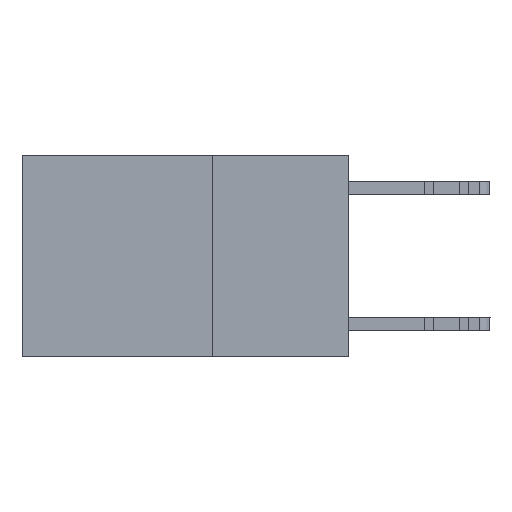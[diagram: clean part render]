
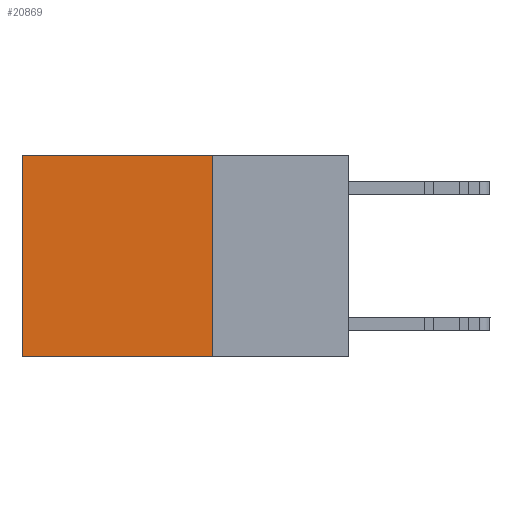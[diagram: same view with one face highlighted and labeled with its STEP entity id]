
A CAD part, left-side view. The second image highlights one B-rep face of the part: STEP entity #20869.
In plain terms, the highlighted planar face has unit normal (-1, 0, 0).
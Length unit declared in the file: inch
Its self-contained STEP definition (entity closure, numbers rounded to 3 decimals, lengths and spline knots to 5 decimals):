
#2307 = DIRECTION ( 'NONE',  ( 0., 0., -1. ) ) ;
#2940 = VECTOR ( 'NONE', #20422, 39.37008 ) ;
#3790 = LINE ( 'NONE', #25389, #2940 ) ;
#4039 = EDGE_CURVE ( 'NONE', #20741, #28897, #4677, .T. ) ;
#4332 = VECTOR ( 'NONE', #23556, 39.37008 ) ;
#4677 = LINE ( 'NONE', #25523, #4332 ) ;
#5005 = CARTESIAN_POINT ( 'NONE',  ( 0.2625, 0.6, -0.37 ) ) ;
#5648 = ORIENTED_EDGE ( 'NONE', *, *, #29035, .T. ) ;
#5797 = EDGE_CURVE ( 'NONE', #12769, #15452, #21283, .T. ) ;
#6502 = CARTESIAN_POINT ( 'NONE',  ( 0.2625, 0.25, 0. ) ) ;
#7311 = DIRECTION ( 'NONE',  ( 0., 0., -1. ) ) ;
#7566 = CARTESIAN_POINT ( 'NONE',  ( 0.2625, 0.25, 0. ) ) ;
#8983 = EDGE_CURVE ( 'NONE', #15452, #28897, #22191, .T. ) ;
#11706 = FACE_OUTER_BOUND ( 'NONE', #30115, .T. ) ;
#12769 = VERTEX_POINT ( 'NONE', #6502 ) ;
#14341 = CARTESIAN_POINT ( 'NONE',  ( 0.2625, 0.6, 0. ) ) ;
#14862 = DIRECTION ( 'NONE',  ( 0., 1., 0. ) ) ;
#14876 = PLANE ( 'NONE',  #24921 ) ;
#15012 = ORIENTED_EDGE ( 'NONE', *, *, #4039, .T. ) ;
#15452 = VERTEX_POINT ( 'NONE', #20140 ) ;
#15571 = CARTESIAN_POINT ( 'NONE',  ( 0.2625, 0.25, -0.37 ) ) ;
#17368 = DIRECTION ( 'NONE',  ( 1., 0., 0. ) ) ;
#18690 = ORIENTED_EDGE ( 'NONE', *, *, #8983, .F. ) ;
#19443 = ORIENTED_EDGE ( 'NONE', *, *, #5797, .F. ) ;
#20140 = CARTESIAN_POINT ( 'NONE',  ( 0.2625, 0.25, -0.37 ) ) ;
#20422 = DIRECTION ( 'NONE',  ( 0., 1., 0. ) ) ;
#20741 = VERTEX_POINT ( 'NONE', #14341 ) ;
#20869 = ADVANCED_FACE ( 'NONE', ( #11706 ), #14876, .F. ) ;
#21241 = VECTOR ( 'NONE', #7311, 39.37008 ) ;
#21283 = LINE ( 'NONE', #7566, #21241 ) ;
#22031 = VECTOR ( 'NONE', #14862, 39.37008 ) ;
#22191 = LINE ( 'NONE', #15571, #22031 ) ;
#23556 = DIRECTION ( 'NONE',  ( 0., 0., -1. ) ) ;
#24921 = AXIS2_PLACEMENT_3D ( 'NONE', #31996, #17368, #2307 ) ;
#25389 = CARTESIAN_POINT ( 'NONE',  ( 0.2625, 0.25, 0. ) ) ;
#25523 = CARTESIAN_POINT ( 'NONE',  ( 0.2625, 0.6, 0. ) ) ;
#28897 = VERTEX_POINT ( 'NONE', #5005 ) ;
#29035 = EDGE_CURVE ( 'NONE', #12769, #20741, #3790, .T. ) ;
#30115 = EDGE_LOOP ( 'NONE', ( #15012, #18690, #19443, #5648 ) ) ;
#31996 = CARTESIAN_POINT ( 'NONE',  ( 0.2625, 0.25, 0. ) ) ;
